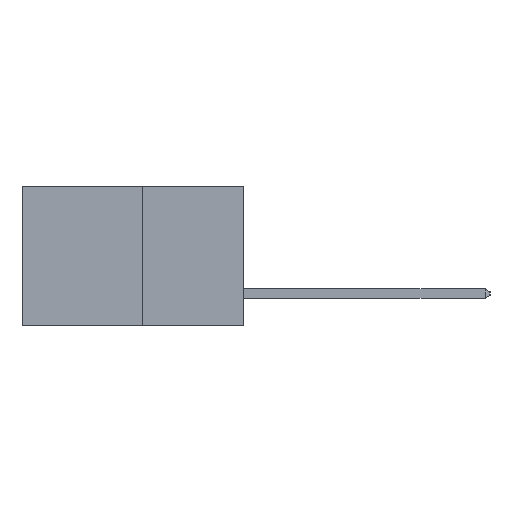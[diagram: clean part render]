
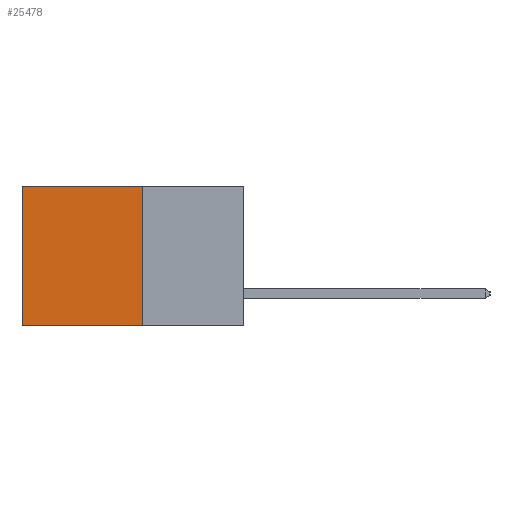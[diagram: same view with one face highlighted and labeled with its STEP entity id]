
A CAD part, left-side view. The second image highlights one B-rep face of the part: STEP entity #25478.
In plain terms, the highlighted planar face has unit normal (-1, 0, 0).
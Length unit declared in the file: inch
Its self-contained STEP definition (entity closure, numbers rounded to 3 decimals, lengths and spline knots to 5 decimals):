
#1034 = EDGE_CURVE ( 'NONE', #5559, #18000, #22101, .T. ) ;
#1630 = LINE ( 'NONE', #24075, #24761 ) ;
#1666 = CARTESIAN_POINT ( 'NONE',  ( 0.277, 0.27, 0. ) ) ;
#2817 = VECTOR ( 'NONE', #20875, 39.37008 ) ;
#3668 = PLANE ( 'NONE',  #8185 ) ;
#4198 = VERTEX_POINT ( 'NONE', #17737 ) ;
#5559 = VERTEX_POINT ( 'NONE', #1666 ) ;
#6051 = DIRECTION ( 'NONE',  ( 1., 0., 0. ) ) ;
#6287 = VECTOR ( 'NONE', #23486, 39.37008 ) ;
#6479 = ORIENTED_EDGE ( 'NONE', *, *, #17262, .F. ) ;
#7848 = CARTESIAN_POINT ( 'NONE',  ( 0.277, 0.27, -0.37 ) ) ;
#8185 = AXIS2_PLACEMENT_3D ( 'NONE', #19546, #6051, #21685 ) ;
#8417 = ORIENTED_EDGE ( 'NONE', *, *, #1034, .F. ) ;
#10691 = ORIENTED_EDGE ( 'NONE', *, *, #14612, .T. ) ;
#10826 = DIRECTION ( 'NONE',  ( 0., 0., -1. ) ) ;
#11026 = EDGE_CURVE ( 'NONE', #26236, #4198, #1630, .T. ) ;
#12270 = ORIENTED_EDGE ( 'NONE', *, *, #11026, .T. ) ;
#12366 = LINE ( 'NONE', #7848, #6287 ) ;
#13748 = EDGE_LOOP ( 'NONE', ( #12270, #6479, #8417, #10691 ) ) ;
#14612 = EDGE_CURVE ( 'NONE', #5559, #26236, #16056, .T. ) ;
#14650 = VECTOR ( 'NONE', #17590, 39.37008 ) ;
#15121 = CARTESIAN_POINT ( 'NONE',  ( 0.277, 0.27, -0.37 ) ) ;
#16056 = LINE ( 'NONE', #26216, #14650 ) ;
#17262 = EDGE_CURVE ( 'NONE', #18000, #4198, #12366, .T. ) ;
#17590 = DIRECTION ( 'NONE',  ( 0., 1., 0. ) ) ;
#17737 = CARTESIAN_POINT ( 'NONE',  ( 0.277, 0.59, -0.37 ) ) ;
#18000 = VERTEX_POINT ( 'NONE', #15121 ) ;
#18138 = CARTESIAN_POINT ( 'NONE',  ( 0.277, 0.27, -0.37 ) ) ;
#19546 = CARTESIAN_POINT ( 'NONE',  ( 0.277, 0.27, -0.37 ) ) ;
#20875 = DIRECTION ( 'NONE',  ( 0., 0., -1. ) ) ;
#21685 = DIRECTION ( 'NONE',  ( 0., 0., -1. ) ) ;
#22101 = LINE ( 'NONE', #18138, #2817 ) ;
#23486 = DIRECTION ( 'NONE',  ( 0., 1., 0. ) ) ;
#24075 = CARTESIAN_POINT ( 'NONE',  ( 0.277, 0.59, -0.37 ) ) ;
#24745 = CARTESIAN_POINT ( 'NONE',  ( 0.277, 0.59, 0. ) ) ;
#24761 = VECTOR ( 'NONE', #10826, 39.37008 ) ;
#25478 = ADVANCED_FACE ( 'NONE', ( #26815 ), #3668, .F. ) ;
#26216 = CARTESIAN_POINT ( 'NONE',  ( 0.277, 0.27, 0. ) ) ;
#26236 = VERTEX_POINT ( 'NONE', #24745 ) ;
#26815 = FACE_OUTER_BOUND ( 'NONE', #13748, .T. ) ;
